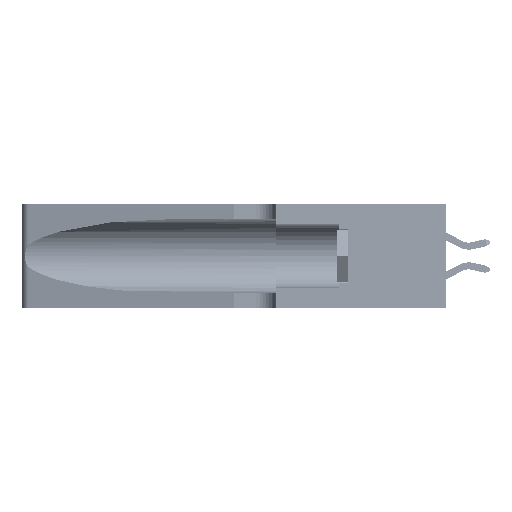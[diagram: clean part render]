
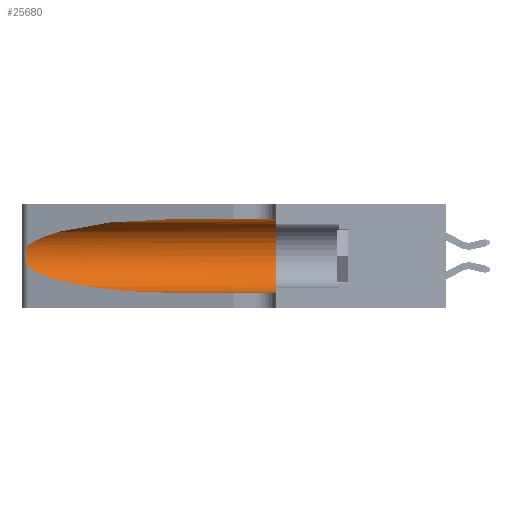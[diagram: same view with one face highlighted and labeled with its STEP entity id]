
A CAD part, left-side view. The second image highlights one B-rep face of the part: STEP entity #25680.
In plain terms, the highlighted cylindrical face has radius 3.308 mm (diameter 6.617 mm), a partial arc.
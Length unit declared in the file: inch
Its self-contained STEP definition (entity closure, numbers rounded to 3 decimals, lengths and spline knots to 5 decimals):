
#2270 = CARTESIAN_POINT ( 'NONE',  ( 0.1305, 0.35, 0.185 ) ) ;
#2539 = ORIENTED_EDGE ( 'NONE', *, *, #31274, .T. ) ;
#2631 = CARTESIAN_POINT ( 'NONE',  ( 0.25487, 1.22718, 0.22369 ) ) ;
#3135 = CARTESIAN_POINT ( 'NONE',  ( 0.25555, 1.22993, 0.14849 ) ) ;
#3307 = B_SPLINE_CURVE_WITH_KNOTS ( 'NONE', 3,
 ( #2631, #19097, #3726, #12230, #23597, #38539, #28328, #38935, #6724, #50693, #6509, #26503, #3135, #15209 ),
 .UNSPECIFIED., .F., .F.,
 ( 4, 2, 2, 2, 2, 2, 4 ),
 ( 0., 0.00027, 0.00053, 0.00107, 0.0016, 0.00187, 0.00214 ),
 .UNSPECIFIED. ) ;
#3726 = CARTESIAN_POINT ( 'NONE',  ( 0.25639, 1.23184, 0.21858 ) ) ;
#3958 = EDGE_CURVE ( 'NONE', #39444, #41697, #3307, .T. ) ;
#4671 = CARTESIAN_POINT ( 'NONE',  ( 0.2373, 1.15595, 0.28018 ) ) ;
#6509 = CARTESIAN_POINT ( 'NONE',  ( 0.25789, 1.23486, 0.15765 ) ) ;
#6577 = VECTOR ( 'NONE', #32712, 39.37008 ) ;
#6724 = CARTESIAN_POINT ( 'NONE',  ( 0.26017, 1.23833, 0.17102 ) ) ;
#7755 = AXIS2_PLACEMENT_3D ( 'NONE', #47040, #23483, #27762 ) ;
#7949 = CIRCLE ( 'NONE', #49025, 0.13025 ) ;
#8416 = LINE ( 'NONE', #37200, #6577 ) ;
#8697 = CARTESIAN_POINT ( 'NONE',  ( 0.25487, 1.22718, 0.22369 ) ) ;
#9949 = LINE ( 'NONE', #48807, #25985 ) ;
#10303 =( BOUNDED_CURVE ( )  B_SPLINE_CURVE ( 3, ( #47804, #12451, #4671, #8697 ),
 .UNSPECIFIED., .F., .F. ) 
 B_SPLINE_CURVE_WITH_KNOTS ( ( 4, 4 ),
 ( 1.5708, 2.84003 ),
 .UNSPECIFIED. ) 
 CURVE ( )  GEOMETRIC_REPRESENTATION_ITEM ( )  RATIONAL_B_SPLINE_CURVE ( ( 1., 0.87, 0.87, 1. ) ) 
 REPRESENTATION_ITEM ( '' )  );
#11102 = CARTESIAN_POINT ( 'NONE',  ( 0.2373, 1.15595, 0.08982 ) ) ;
#12230 = CARTESIAN_POINT ( 'NONE',  ( 0.25787, 1.23484, 0.2124 ) ) ;
#12451 = CARTESIAN_POINT ( 'NONE',  ( 0.18966, 0.96281, 0.31525 ) ) ;
#14694 = CARTESIAN_POINT ( 'NONE',  ( 0.1305, 0.72297, 0.05475 ) ) ;
#15209 = CARTESIAN_POINT ( 'NONE',  ( 0.25487, 1.22718, 0.14631 ) ) ;
#15352 = DIRECTION ( 'NONE',  ( 0., 1., 0. ) ) ;
#18132 = DIRECTION ( 'NONE',  ( 0., -1., 0. ) ) ;
#18410 = EDGE_LOOP ( 'NONE', ( #35964, #18642, #2539, #19827, #21049, #21492 ) ) ;
#18642 = ORIENTED_EDGE ( 'NONE', *, *, #3958, .T. ) ;
#19097 = CARTESIAN_POINT ( 'NONE',  ( 0.25555, 1.22994, 0.2215 ) ) ;
#19827 = ORIENTED_EDGE ( 'NONE', *, *, #38907, .T. ) ;
#19829 = CARTESIAN_POINT ( 'NONE',  ( 0.1305, 0.35, 0.05475 ) ) ;
#20899 = EDGE_CURVE ( 'NONE', #29839, #35081, #9949, .T. ) ;
#21049 = ORIENTED_EDGE ( 'NONE', *, *, #26180, .F. ) ;
#21492 = ORIENTED_EDGE ( 'NONE', *, *, #20899, .F. ) ;
#22969 = CARTESIAN_POINT ( 'NONE',  ( 0.25487, 1.22718, 0.14631 ) ) ;
#23483 = DIRECTION ( 'NONE',  ( 0., -1., 0. ) ) ;
#23597 = CARTESIAN_POINT ( 'NONE',  ( 0.25854, 1.2359, 0.20912 ) ) ;
#25680 = ADVANCED_FACE ( 'NONE', ( #37025 ), #42528, .F. ) ;
#25985 = VECTOR ( 'NONE', #18132, 39.37008 ) ;
#26180 = EDGE_CURVE ( 'NONE', #35081, #47592, #7949, .T. ) ;
#26379 = CARTESIAN_POINT ( 'NONE',  ( 0.1305, 0.35, 0.31525 ) ) ;
#26503 = CARTESIAN_POINT ( 'NONE',  ( 0.25639, 1.23186, 0.15144 ) ) ;
#27762 = DIRECTION ( 'NONE',  ( 0., 0., -1. ) ) ;
#28328 = CARTESIAN_POINT ( 'NONE',  ( 0.26075, 1.23896, 0.19203 ) ) ;
#29598 = EDGE_CURVE ( 'NONE', #29839, #39444, #10303, .T. ) ;
#29839 = VERTEX_POINT ( 'NONE', #30363 ) ;
#30363 = CARTESIAN_POINT ( 'NONE',  ( 0.1305, 0.72297, 0.31525 ) ) ;
#31205 = VERTEX_POINT ( 'NONE', #14694 ) ;
#31274 = EDGE_CURVE ( 'NONE', #41697, #31205, #33981, .T. ) ;
#32712 = DIRECTION ( 'NONE',  ( 0., -1., 0. ) ) ;
#33796 = DIRECTION ( 'NONE',  ( 0., 0., 1. ) ) ;
#33981 =( BOUNDED_CURVE ( )  B_SPLINE_CURVE ( 3, ( #34662, #11102, #42119, #38664 ),
 .UNSPECIFIED., .F., .F. ) 
 B_SPLINE_CURVE_WITH_KNOTS ( ( 4, 4 ),
 ( 3.44316, 4.71239 ),
 .UNSPECIFIED. ) 
 CURVE ( )  GEOMETRIC_REPRESENTATION_ITEM ( )  RATIONAL_B_SPLINE_CURVE ( ( 1., 0.87, 0.87, 1. ) ) 
 REPRESENTATION_ITEM ( '' )  );
#34662 = CARTESIAN_POINT ( 'NONE',  ( 0.25487, 1.22718, 0.14631 ) ) ;
#35081 = VERTEX_POINT ( 'NONE', #26379 ) ;
#35964 = ORIENTED_EDGE ( 'NONE', *, *, #29598, .T. ) ;
#37025 = FACE_OUTER_BOUND ( 'NONE', #18410, .T. ) ;
#37200 = CARTESIAN_POINT ( 'NONE',  ( 0.1305, 1.61858, 0.05475 ) ) ;
#38539 = CARTESIAN_POINT ( 'NONE',  ( 0.26018, 1.23835, 0.19895 ) ) ;
#38664 = CARTESIAN_POINT ( 'NONE',  ( 0.1305, 0.72297, 0.05475 ) ) ;
#38907 = EDGE_CURVE ( 'NONE', #31205, #47592, #8416, .T. ) ;
#38935 = CARTESIAN_POINT ( 'NONE',  ( 0.26075, 1.23896, 0.178 ) ) ;
#39444 = VERTEX_POINT ( 'NONE', #44183 ) ;
#41697 = VERTEX_POINT ( 'NONE', #22969 ) ;
#42119 = CARTESIAN_POINT ( 'NONE',  ( 0.18966, 0.96281, 0.05475 ) ) ;
#42528 = CYLINDRICAL_SURFACE ( 'NONE', #7755, 0.13025 ) ;
#44183 = CARTESIAN_POINT ( 'NONE',  ( 0.25487, 1.22718, 0.22369 ) ) ;
#47040 = CARTESIAN_POINT ( 'NONE',  ( 0.1305, 1.61858, 0.185 ) ) ;
#47592 = VERTEX_POINT ( 'NONE', #19829 ) ;
#47804 = CARTESIAN_POINT ( 'NONE',  ( 0.1305, 0.72297, 0.31525 ) ) ;
#48807 = CARTESIAN_POINT ( 'NONE',  ( 0.1305, 1.61858, 0.31525 ) ) ;
#49025 = AXIS2_PLACEMENT_3D ( 'NONE', #2270, #15352, #33796 ) ;
#50693 = CARTESIAN_POINT ( 'NONE',  ( 0.25856, 1.23593, 0.16098 ) ) ;
